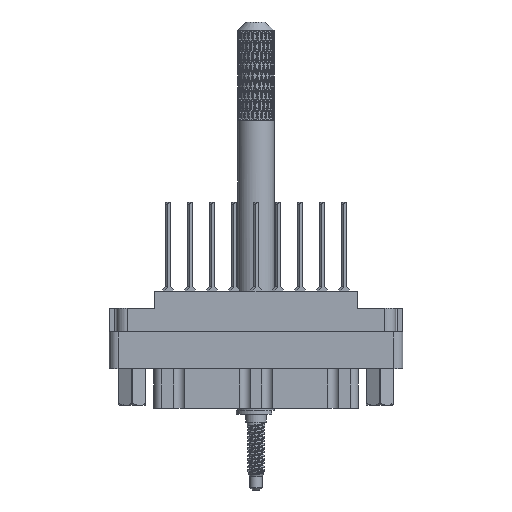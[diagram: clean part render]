
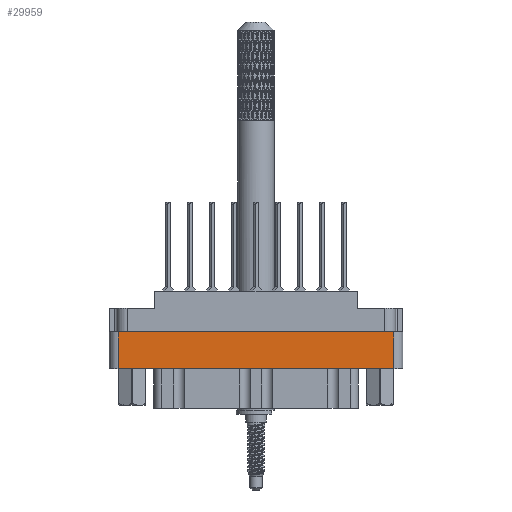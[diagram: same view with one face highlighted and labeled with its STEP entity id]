
A CAD part, front view. The second image highlights one B-rep face of the part: STEP entity #29959.
In plain terms, the highlighted planar face has unit normal (0, -1, 0).
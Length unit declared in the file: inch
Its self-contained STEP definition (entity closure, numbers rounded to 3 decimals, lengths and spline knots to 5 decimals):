
#2468 = VERTEX_POINT ( 'NONE', #35602 ) ;
#3105 = VECTOR ( 'NONE', #5093, 39.37008 ) ;
#5093 = DIRECTION ( 'NONE',  ( 0., 0., 1. ) ) ;
#6833 = EDGE_LOOP ( 'NONE', ( #99065, #40335, #38922, #32606 ) ) ;
#7665 = VERTEX_POINT ( 'NONE', #105178 ) ;
#10395 = CARTESIAN_POINT ( 'NONE',  ( 0.938, -0.438, -0.277 ) ) ;
#13095 = DIRECTION ( 'NONE',  ( 0., 0., 1. ) ) ;
#14176 = DIRECTION ( 'NONE',  ( -1., 0., 0. ) ) ;
#20909 = CARTESIAN_POINT ( 'NONE',  ( 0.938, -0.438, -0.529 ) ) ;
#26536 = VECTOR ( 'NONE', #14176, 39.37008 ) ;
#29959 = ADVANCED_FACE ( 'NONE', ( #102584 ), #43185, .T. ) ;
#32606 = ORIENTED_EDGE ( 'NONE', *, *, #66872, .F. ) ;
#35602 = CARTESIAN_POINT ( 'NONE',  ( -0.938, -0.438, -0.277 ) ) ;
#38922 = ORIENTED_EDGE ( 'NONE', *, *, #67351, .T. ) ;
#40335 = ORIENTED_EDGE ( 'NONE', *, *, #80614, .F. ) ;
#42613 = CARTESIAN_POINT ( 'NONE',  ( -1., -0.438, -0.277 ) ) ;
#43185 = PLANE ( 'NONE',  #99463 ) ;
#47888 = CARTESIAN_POINT ( 'NONE',  ( 0.938, -0.438, -0.798 ) ) ;
#50686 = EDGE_CURVE ( 'NONE', #70538, #2468, #75728, .T. ) ;
#60611 = DIRECTION ( 'NONE',  ( 0., 0., -1. ) ) ;
#64146 = LINE ( 'NONE', #20909, #26536 ) ;
#66799 = LINE ( 'NONE', #42613, #77573 ) ;
#66872 = EDGE_CURVE ( 'NONE', #2468, #74270, #66799, .T. ) ;
#67351 = EDGE_CURVE ( 'NONE', #7665, #74270, #107254, .T. ) ;
#70538 = VERTEX_POINT ( 'NONE', #100430 ) ;
#72120 = VECTOR ( 'NONE', #13095, 39.37008 ) ;
#74270 = VERTEX_POINT ( 'NONE', #10395 ) ;
#75728 = LINE ( 'NONE', #100356, #3105 ) ;
#77573 = VECTOR ( 'NONE', #101456, 39.37008 ) ;
#80614 = EDGE_CURVE ( 'NONE', #7665, #70538, #64146, .T. ) ;
#84170 = CARTESIAN_POINT ( 'NONE',  ( -0.938, -0.438, -0.798 ) ) ;
#93666 = DIRECTION ( 'NONE',  ( 0., -1., 0. ) ) ;
#99065 = ORIENTED_EDGE ( 'NONE', *, *, #50686, .F. ) ;
#99463 = AXIS2_PLACEMENT_3D ( 'NONE', #84170, #93666, #60611 ) ;
#100356 = CARTESIAN_POINT ( 'NONE',  ( -0.938, -0.438, -0.798 ) ) ;
#100430 = CARTESIAN_POINT ( 'NONE',  ( -0.938, -0.438, -0.529 ) ) ;
#101456 = DIRECTION ( 'NONE',  ( 1., 0., 0. ) ) ;
#102584 = FACE_OUTER_BOUND ( 'NONE', #6833, .T. ) ;
#105178 = CARTESIAN_POINT ( 'NONE',  ( 0.938, -0.438, -0.529 ) ) ;
#107254 = LINE ( 'NONE', #47888, #72120 ) ;
